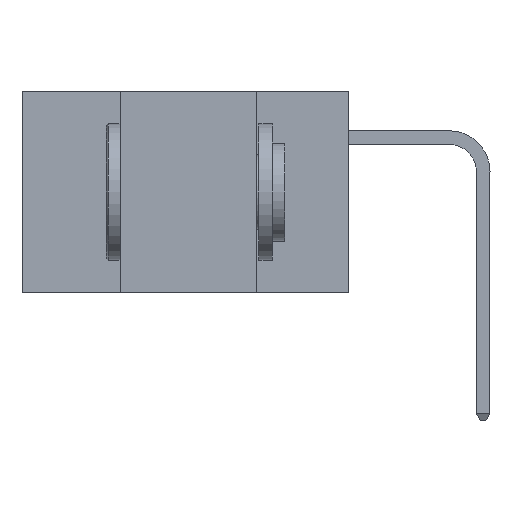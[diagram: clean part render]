
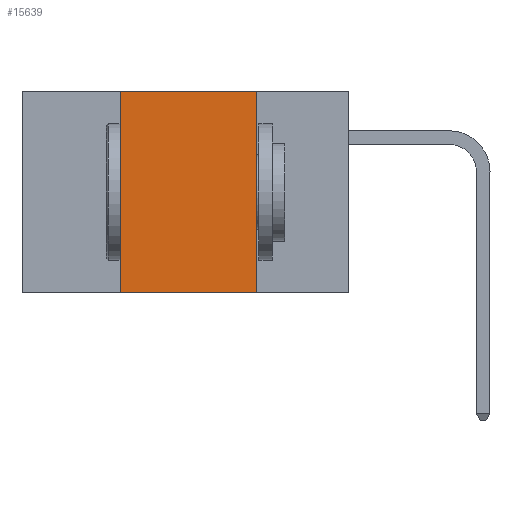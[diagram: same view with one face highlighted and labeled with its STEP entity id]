
A CAD part, left-side view. The second image highlights one B-rep face of the part: STEP entity #15639.
In plain terms, the highlighted planar face has unit normal (-1, 0, 0).
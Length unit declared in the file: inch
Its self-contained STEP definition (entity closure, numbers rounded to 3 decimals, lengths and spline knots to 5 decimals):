
#8 = EDGE_LOOP ( 'NONE', ( #26791, #8434, #13018, #17954 ) ) ;
#443 = DIRECTION ( 'NONE',  ( 0., -1., 0. ) ) ;
#893 = VECTOR ( 'NONE', #1057, 39.37008 ) ;
#1057 = DIRECTION ( 'NONE',  ( 0., 0., -1. ) ) ;
#1118 = VERTEX_POINT ( 'NONE', #3547 ) ;
#1464 = VECTOR ( 'NONE', #26621, 39.37008 ) ;
#1712 = VERTEX_POINT ( 'NONE', #18941 ) ;
#2700 = EDGE_CURVE ( 'NONE', #1712, #17313, #7613, .T. ) ;
#3547 = CARTESIAN_POINT ( 'NONE',  ( 0., 0.17, 0. ) ) ;
#3645 = VECTOR ( 'NONE', #443, 39.37008 ) ;
#5715 = LINE ( 'NONE', #29113, #893 ) ;
#6851 = AXIS2_PLACEMENT_3D ( 'NONE', #10740, #13352, #13469 ) ;
#6939 = DIRECTION ( 'NONE',  ( 0., 0., 1. ) ) ;
#7089 = FACE_OUTER_BOUND ( 'NONE', #8, .T. ) ;
#7613 = LINE ( 'NONE', #28185, #3645 ) ;
#7756 = CARTESIAN_POINT ( 'NONE',  ( 0., 0.17, -0.37 ) ) ;
#8434 = ORIENTED_EDGE ( 'NONE', *, *, #15807, .F. ) ;
#8658 = CARTESIAN_POINT ( 'NONE',  ( 0., 0.42, 0. ) ) ;
#10740 = CARTESIAN_POINT ( 'NONE',  ( 0., 0.6, 0. ) ) ;
#10856 = PLANE ( 'NONE',  #6851 ) ;
#11778 = LINE ( 'NONE', #29858, #19426 ) ;
#12668 = EDGE_CURVE ( 'NONE', #1712, #19418, #11778, .T. ) ;
#13018 = ORIENTED_EDGE ( 'NONE', *, *, #12668, .F. ) ;
#13352 = DIRECTION ( 'NONE',  ( 1., 0., 0. ) ) ;
#13469 = DIRECTION ( 'NONE',  ( 0., 0., -1. ) ) ;
#13625 = EDGE_CURVE ( 'NONE', #1118, #17313, #5715, .T. ) ;
#15094 = LINE ( 'NONE', #18944, #1464 ) ;
#15639 = ADVANCED_FACE ( 'NONE', ( #7089 ), #10856, .F. ) ;
#15807 = EDGE_CURVE ( 'NONE', #19418, #1118, #15094, .T. ) ;
#17313 = VERTEX_POINT ( 'NONE', #7756 ) ;
#17954 = ORIENTED_EDGE ( 'NONE', *, *, #2700, .T. ) ;
#18941 = CARTESIAN_POINT ( 'NONE',  ( 0., 0.42, -0.37 ) ) ;
#18944 = CARTESIAN_POINT ( 'NONE',  ( 0., 0.6, 0. ) ) ;
#19418 = VERTEX_POINT ( 'NONE', #8658 ) ;
#19426 = VECTOR ( 'NONE', #6939, 39.37008 ) ;
#26621 = DIRECTION ( 'NONE',  ( 0., -1., 0. ) ) ;
#26791 = ORIENTED_EDGE ( 'NONE', *, *, #13625, .F. ) ;
#28185 = CARTESIAN_POINT ( 'NONE',  ( 0., 0.6, -0.37 ) ) ;
#29113 = CARTESIAN_POINT ( 'NONE',  ( 0., 0.17, 0. ) ) ;
#29858 = CARTESIAN_POINT ( 'NONE',  ( 0., 0.42, 0. ) ) ;
